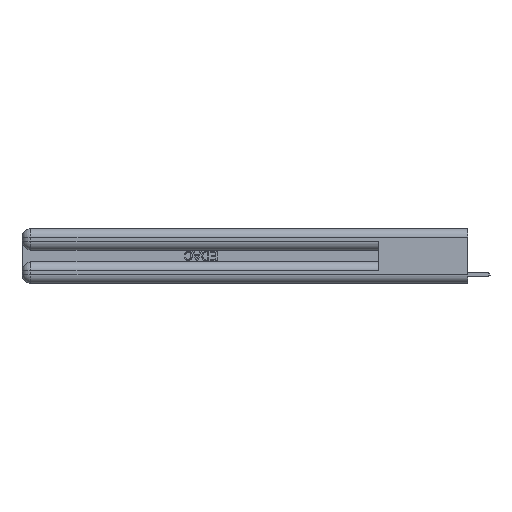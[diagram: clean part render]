
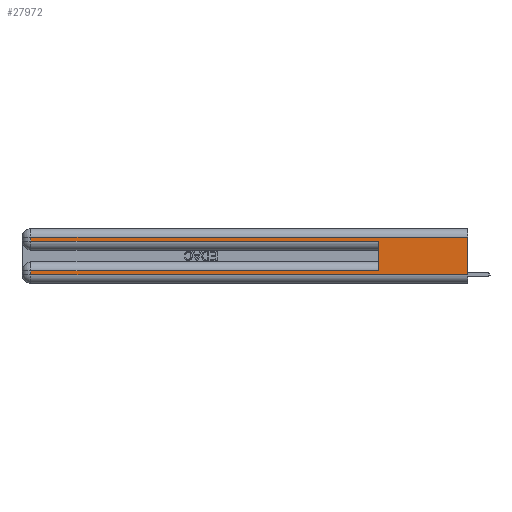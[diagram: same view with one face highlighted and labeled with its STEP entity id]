
A CAD part, left-side view. The second image highlights one B-rep face of the part: STEP entity #27972.
In plain terms, the highlighted planar face has unit normal (-1, 0, 0).
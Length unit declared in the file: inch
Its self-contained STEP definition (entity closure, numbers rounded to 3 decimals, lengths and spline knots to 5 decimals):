
#1174 = LINE ( 'NONE', #8486, #12361 ) ;
#1209 = CARTESIAN_POINT ( 'NONE',  ( 0., 0.6, 0.085 ) ) ;
#1282 = CARTESIAN_POINT ( 'NONE',  ( 0., 0., 0.06 ) ) ;
#2088 = EDGE_CURVE ( 'NONE', #14341, #21488, #11879, .T. ) ;
#2119 = EDGE_CURVE ( 'NONE', #5017, #4256, #21336, .T. ) ;
#2851 = ORIENTED_EDGE ( 'NONE', *, *, #17606, .F. ) ;
#2992 = EDGE_CURVE ( 'NONE', #29197, #14325, #20980, .T. ) ;
#3407 = CARTESIAN_POINT ( 'NONE',  ( 0., 0., 0.06 ) ) ;
#4032 = LINE ( 'NONE', #3407, #28017 ) ;
#4101 = ORIENTED_EDGE ( 'NONE', *, *, #14424, .T. ) ;
#4256 = VERTEX_POINT ( 'NONE', #18715 ) ;
#4286 = VERTEX_POINT ( 'NONE', #11277 ) ;
#4979 = EDGE_CURVE ( 'NONE', #14325, #4286, #18297, .T. ) ;
#5017 = VERTEX_POINT ( 'NONE', #1209 ) ;
#5638 = EDGE_LOOP ( 'NONE', ( #2851, #11131, #27926, #6810, #16101, #4101, #19350, #14804 ) ) ;
#5801 = VECTOR ( 'NONE', #13487, 39.37008 ) ;
#6399 = CARTESIAN_POINT ( 'NONE',  ( 0., 2.94, 0.085 ) ) ;
#6718 = LINE ( 'NONE', #28154, #7193 ) ;
#6810 = ORIENTED_EDGE ( 'NONE', *, *, #8873, .T. ) ;
#7070 = CARTESIAN_POINT ( 'NONE',  ( 0., 0.6, 0.145 ) ) ;
#7193 = VECTOR ( 'NONE', #16185, 39.37008 ) ;
#8486 = CARTESIAN_POINT ( 'NONE',  ( 0., 0., 0.285 ) ) ;
#8873 = EDGE_CURVE ( 'NONE', #4286, #4256, #1174, .T. ) ;
#10069 = PLANE ( 'NONE',  #19124 ) ;
#11131 = ORIENTED_EDGE ( 'NONE', *, *, #2992, .T. ) ;
#11172 = CARTESIAN_POINT ( 'NONE',  ( 0., 2.94, 0.37 ) ) ;
#11277 = CARTESIAN_POINT ( 'NONE',  ( 0., 2.94, 0.285 ) ) ;
#11879 = LINE ( 'NONE', #18875, #12221 ) ;
#12221 = VECTOR ( 'NONE', #13905, 39.37008 ) ;
#12361 = VECTOR ( 'NONE', #17955, 39.37008 ) ;
#13487 = DIRECTION ( 'NONE',  ( 0., 0., -1. ) ) ;
#13905 = DIRECTION ( 'NONE',  ( 0., 0., -1. ) ) ;
#14325 = VERTEX_POINT ( 'NONE', #14946 ) ;
#14341 = VERTEX_POINT ( 'NONE', #6399 ) ;
#14424 = EDGE_CURVE ( 'NONE', #5017, #14341, #24514, .T. ) ;
#14576 = DIRECTION ( 'NONE',  ( 0., 1., 0. ) ) ;
#14804 = ORIENTED_EDGE ( 'NONE', *, *, #26938, .T. ) ;
#14946 = CARTESIAN_POINT ( 'NONE',  ( 0., 2.94, 0.31 ) ) ;
#15010 = DIRECTION ( 'NONE',  ( 1., 0., 0. ) ) ;
#15157 = DIRECTION ( 'NONE',  ( 0., 0., -1. ) ) ;
#16101 = ORIENTED_EDGE ( 'NONE', *, *, #2119, .F. ) ;
#16185 = DIRECTION ( 'NONE',  ( 0., 0., -1. ) ) ;
#17060 = CARTESIAN_POINT ( 'NONE',  ( 0., 0., 0.085 ) ) ;
#17606 = EDGE_CURVE ( 'NONE', #29197, #27191, #6718, .T. ) ;
#17955 = DIRECTION ( 'NONE',  ( 0., -1., 0. ) ) ;
#18169 = DIRECTION ( 'NONE',  ( 0., -1., 0. ) ) ;
#18297 = LINE ( 'NONE', #11172, #5801 ) ;
#18657 = DIRECTION ( 'NONE',  ( 0., 1., 0. ) ) ;
#18715 = CARTESIAN_POINT ( 'NONE',  ( 0., 0.6, 0.285 ) ) ;
#18875 = CARTESIAN_POINT ( 'NONE',  ( 0., 2.94, 0.37 ) ) ;
#19124 = AXIS2_PLACEMENT_3D ( 'NONE', #24803, #15010, #15157 ) ;
#19350 = ORIENTED_EDGE ( 'NONE', *, *, #2088, .T. ) ;
#19814 = FACE_OUTER_BOUND ( 'NONE', #5638, .T. ) ;
#20819 = CARTESIAN_POINT ( 'NONE',  ( 0., 0., 0.31 ) ) ;
#20934 = VECTOR ( 'NONE', #14576, 39.37008 ) ;
#20980 = LINE ( 'NONE', #20819, #28352 ) ;
#21336 = LINE ( 'NONE', #7070, #24130 ) ;
#21345 = CARTESIAN_POINT ( 'NONE',  ( 0., 2.94, 0.06 ) ) ;
#21488 = VERTEX_POINT ( 'NONE', #21345 ) ;
#23375 = DIRECTION ( 'NONE',  ( 0., 0., 1. ) ) ;
#23610 = CARTESIAN_POINT ( 'NONE',  ( 0., 0., 0.31 ) ) ;
#24130 = VECTOR ( 'NONE', #23375, 39.37008 ) ;
#24514 = LINE ( 'NONE', #17060, #20934 ) ;
#24803 = CARTESIAN_POINT ( 'NONE',  ( 0., 0., 0.37 ) ) ;
#26938 = EDGE_CURVE ( 'NONE', #21488, #27191, #4032, .T. ) ;
#27191 = VERTEX_POINT ( 'NONE', #1282 ) ;
#27926 = ORIENTED_EDGE ( 'NONE', *, *, #4979, .T. ) ;
#27972 = ADVANCED_FACE ( 'NONE', ( #19814 ), #10069, .F. ) ;
#28017 = VECTOR ( 'NONE', #18169, 39.37008 ) ;
#28154 = CARTESIAN_POINT ( 'NONE',  ( 0., 0., 0.37 ) ) ;
#28352 = VECTOR ( 'NONE', #18657, 39.37008 ) ;
#29197 = VERTEX_POINT ( 'NONE', #23610 ) ;
